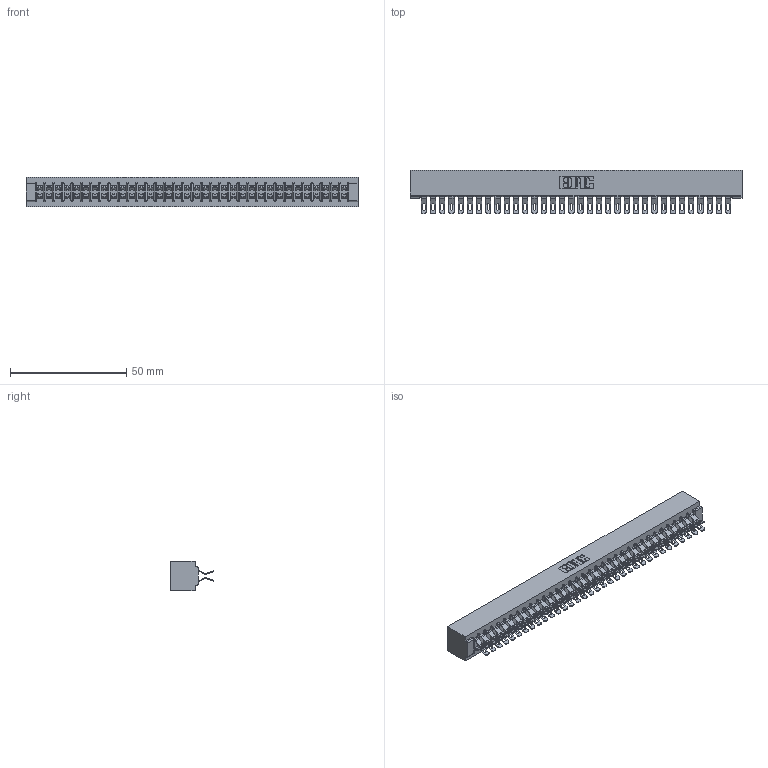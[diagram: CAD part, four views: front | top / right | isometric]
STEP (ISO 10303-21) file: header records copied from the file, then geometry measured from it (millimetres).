
FILE_DESCRIPTION (( 'STEP AP203' ), '1' );
FILE_NAME ('357-068-555-201.STEP', '2018-08-12T18:08:01', ( '' ), ( '' ), 'SwSTEP 2.0', 'SolidWorks 2016', '' );
FILE_SCHEMA (( 'CONFIG_CONTROL_DESIGN' ));
Length unit declared in the file: inch
Products named in the file (3): 307 Part_No Mounting Lugs; 307-290-001_555; 357-068-555-201
Assembly tree (69 placements, depth 2):
  357-068-555-201
    307 Part_No Mounting Lugs
    307-290-001_555  x68
Bounding box: 142.6 x 18.75 x 12.7 mm (x, y, z)
Volume: 15856.8 mm3; surface area: 20679.7 mm2
Topology: 69 solids, 69 shells, 4293 faces, 12607 edges, 8218 vertices
Faces by surface type: plane 2378, cylinder 1845, sphere 70
Entity records: 31481 total; most frequent: CARTESIAN_POINT 5154, ORIENTED_EDGE 5108, DIRECTION 5058, EDGE_CURVE 2554, VECTOR 1946, LINE 1946, VERTEX_POINT 1652, AXIS2_PLACEMENT_3D 1556
